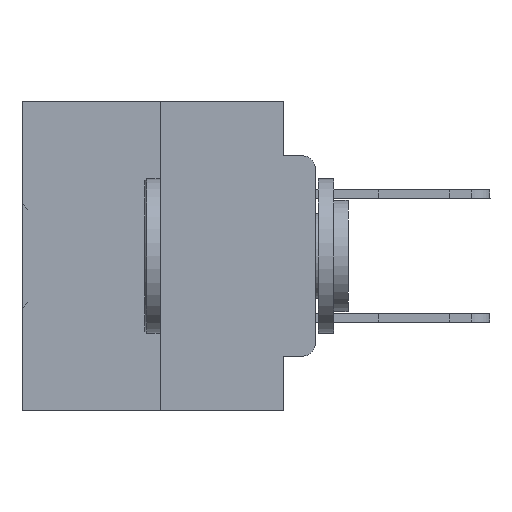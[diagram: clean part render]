
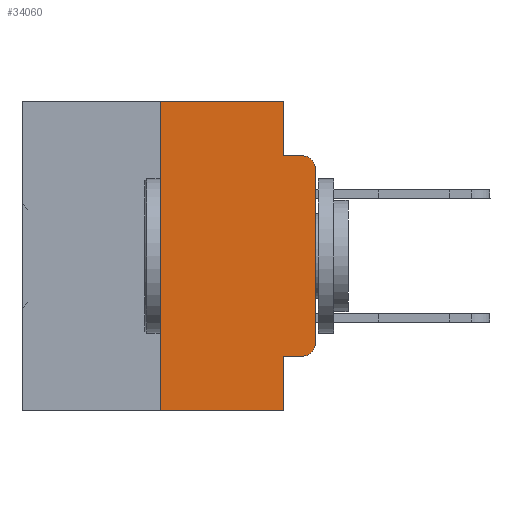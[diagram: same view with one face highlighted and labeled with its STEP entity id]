
A CAD part, left-side view. The second image highlights one B-rep face of the part: STEP entity #34060.
In plain terms, the highlighted planar face has unit normal (-1, 0, 0).
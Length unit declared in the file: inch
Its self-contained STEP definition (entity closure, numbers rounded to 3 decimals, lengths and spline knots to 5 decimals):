
#124 = VECTOR ( 'NONE', #17086, 39.37008 ) ;
#829 = AXIS2_PLACEMENT_3D ( 'NONE', #2584, #35042, #14429 ) ;
#2143 = LINE ( 'NONE', #10694, #124 ) ;
#2584 = CARTESIAN_POINT ( 'NONE',  ( 0., 0.473, 0. ) ) ;
#2869 = VECTOR ( 'NONE', #3727, 39.37008 ) ;
#3241 = VERTEX_POINT ( 'NONE', #8130 ) ;
#3727 = DIRECTION ( 'NONE',  ( 0., -1., 0. ) ) ;
#4307 = CARTESIAN_POINT ( 'NONE',  ( 0., 0.473, -0.5 ) ) ;
#4803 = DIRECTION ( 'NONE',  ( 0., 0., 1. ) ) ;
#5034 = CARTESIAN_POINT ( 'NONE',  ( 0., 0.25, -0.5 ) ) ;
#5106 = VECTOR ( 'NONE', #12397, 39.37008 ) ;
#5188 = VERTEX_POINT ( 'NONE', #22249 ) ;
#5288 = ORIENTED_EDGE ( 'NONE', *, *, #28708, .F. ) ;
#6385 = DIRECTION ( 'NONE',  ( 0., 0., -1. ) ) ;
#8130 = CARTESIAN_POINT ( 'NONE',  ( 0., 0.02, -0.0885 ) ) ;
#8503 = EDGE_CURVE ( 'NONE', #5188, #21527, #2143, .T. ) ;
#8784 = EDGE_CURVE ( 'NONE', #28893, #37621, #30474, .T. ) ;
#10223 = CARTESIAN_POINT ( 'NONE',  ( 0., 0.051, -0.0885 ) ) ;
#10602 = ORIENTED_EDGE ( 'NONE', *, *, #28664, .F. ) ;
#10617 = CARTESIAN_POINT ( 'NONE',  ( 0., 0.051, -0.0885 ) ) ;
#10694 = CARTESIAN_POINT ( 'NONE',  ( 0., 0.051, 0. ) ) ;
#11015 = ORIENTED_EDGE ( 'NONE', *, *, #13485, .T. ) ;
#11222 = ORIENTED_EDGE ( 'NONE', *, *, #19065, .T. ) ;
#11382 = CARTESIAN_POINT ( 'NONE',  ( 0., 0.25, 0. ) ) ;
#11613 = DIRECTION ( 'NONE',  ( 0., -1., 0. ) ) ;
#12397 = DIRECTION ( 'NONE',  ( 0., 0., 1. ) ) ;
#12696 = VERTEX_POINT ( 'NONE', #12899 ) ;
#12899 = CARTESIAN_POINT ( 'NONE',  ( 0., 0.051, -0.4115 ) ) ;
#12946 = DIRECTION ( 'NONE',  ( 0., -1., 0. ) ) ;
#13412 = ORIENTED_EDGE ( 'NONE', *, *, #8784, .T. ) ;
#13485 = EDGE_CURVE ( 'NONE', #33582, #34039, #15563, .T. ) ;
#13810 = ORIENTED_EDGE ( 'NONE', *, *, #17150, .F. ) ;
#14429 = DIRECTION ( 'NONE',  ( 0., 0., -1. ) ) ;
#14542 = CARTESIAN_POINT ( 'NONE',  ( 0., 0.051, -0.4115 ) ) ;
#14668 = CARTESIAN_POINT ( 'NONE',  ( 0., 0., -0.3915 ) ) ;
#14846 = VECTOR ( 'NONE', #12946, 39.37008 ) ;
#15131 = CARTESIAN_POINT ( 'NONE',  ( 0., 0.25, 0. ) ) ;
#15563 = LINE ( 'NONE', #4307, #2869 ) ;
#16274 = CIRCLE ( 'NONE', #23102, 0.02 ) ;
#16449 = LINE ( 'NONE', #11382, #21720 ) ;
#16624 = CARTESIAN_POINT ( 'NONE',  ( 0., 0.473, 0. ) ) ;
#16833 = DIRECTION ( 'NONE',  ( 0., 0., -1. ) ) ;
#17086 = DIRECTION ( 'NONE',  ( 0., 0., -1. ) ) ;
#17150 = EDGE_CURVE ( 'NONE', #33582, #33381, #16449, .T. ) ;
#17925 = AXIS2_PLACEMENT_3D ( 'NONE', #27754, #30678, #27952 ) ;
#19065 = EDGE_CURVE ( 'NONE', #12696, #30879, #20576, .T. ) ;
#20462 = VECTOR ( 'NONE', #16833, 39.37008 ) ;
#20576 = LINE ( 'NONE', #14542, #31063 ) ;
#21035 = CARTESIAN_POINT ( 'NONE',  ( 0., 0.051, -0.5 ) ) ;
#21169 = CARTESIAN_POINT ( 'NONE',  ( 0., 0.02, -0.1085 ) ) ;
#21527 = VERTEX_POINT ( 'NONE', #10617 ) ;
#21720 = VECTOR ( 'NONE', #4803, 39.37008 ) ;
#22106 = LINE ( 'NONE', #25970, #20462 ) ;
#22249 = CARTESIAN_POINT ( 'NONE',  ( 0., 0.051, 0. ) ) ;
#23102 = AXIS2_PLACEMENT_3D ( 'NONE', #21169, #24069, #6385 ) ;
#23429 = EDGE_LOOP ( 'NONE', ( #13412, #38104, #10602, #33479, #5288, #13810, #11015, #25620, #11222, #31452 ) ) ;
#24069 = DIRECTION ( 'NONE',  ( -1., 0., 0. ) ) ;
#24678 = VECTOR ( 'NONE', #37048, 39.37008 ) ;
#25183 = LINE ( 'NONE', #16624, #24678 ) ;
#25620 = ORIENTED_EDGE ( 'NONE', *, *, #30362, .F. ) ;
#25921 = CARTESIAN_POINT ( 'NONE',  ( 0., 0.02, -0.4115 ) ) ;
#25970 = CARTESIAN_POINT ( 'NONE',  ( 0., 0.051, 0. ) ) ;
#26669 = PLANE ( 'NONE',  #829 ) ;
#27754 = CARTESIAN_POINT ( 'NONE',  ( 0., 0.02, -0.3915 ) ) ;
#27952 = DIRECTION ( 'NONE',  ( 0., 0., -1. ) ) ;
#28664 = EDGE_CURVE ( 'NONE', #21527, #3241, #34332, .T. ) ;
#28708 = EDGE_CURVE ( 'NONE', #33381, #5188, #25183, .T. ) ;
#28893 = VERTEX_POINT ( 'NONE', #14668 ) ;
#29469 = EDGE_CURVE ( 'NONE', #30879, #28893, #30960, .T. ) ;
#30362 = EDGE_CURVE ( 'NONE', #12696, #34039, #22106, .T. ) ;
#30474 = LINE ( 'NONE', #30670, #5106 ) ;
#30670 = CARTESIAN_POINT ( 'NONE',  ( 0., 0., 0. ) ) ;
#30678 = DIRECTION ( 'NONE',  ( -1., 0., 0. ) ) ;
#30879 = VERTEX_POINT ( 'NONE', #25921 ) ;
#30960 = CIRCLE ( 'NONE', #17925, 0.02 ) ;
#31063 = VECTOR ( 'NONE', #11613, 39.37008 ) ;
#31452 = ORIENTED_EDGE ( 'NONE', *, *, #29469, .T. ) ;
#33319 = EDGE_CURVE ( 'NONE', #37621, #3241, #16274, .T. ) ;
#33381 = VERTEX_POINT ( 'NONE', #15131 ) ;
#33479 = ORIENTED_EDGE ( 'NONE', *, *, #8503, .F. ) ;
#33582 = VERTEX_POINT ( 'NONE', #5034 ) ;
#34039 = VERTEX_POINT ( 'NONE', #21035 ) ;
#34060 = ADVANCED_FACE ( 'NONE', ( #38152 ), #26669, .F. ) ;
#34332 = LINE ( 'NONE', #10223, #14846 ) ;
#35042 = DIRECTION ( 'NONE',  ( 1., 0., 0. ) ) ;
#36931 = CARTESIAN_POINT ( 'NONE',  ( 0., 0., -0.1085 ) ) ;
#37048 = DIRECTION ( 'NONE',  ( 0., -1., 0. ) ) ;
#37621 = VERTEX_POINT ( 'NONE', #36931 ) ;
#38104 = ORIENTED_EDGE ( 'NONE', *, *, #33319, .T. ) ;
#38152 = FACE_OUTER_BOUND ( 'NONE', #23429, .T. ) ;
